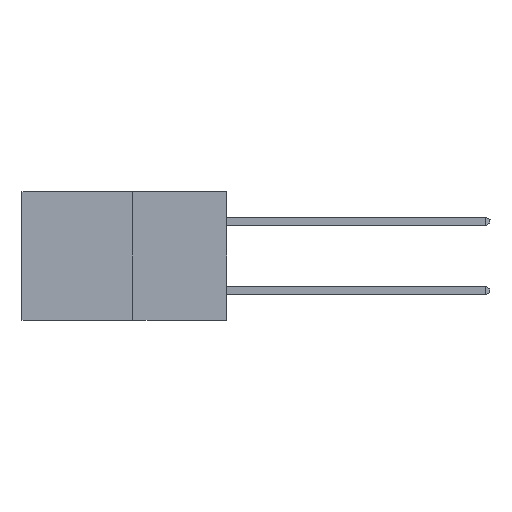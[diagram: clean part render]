
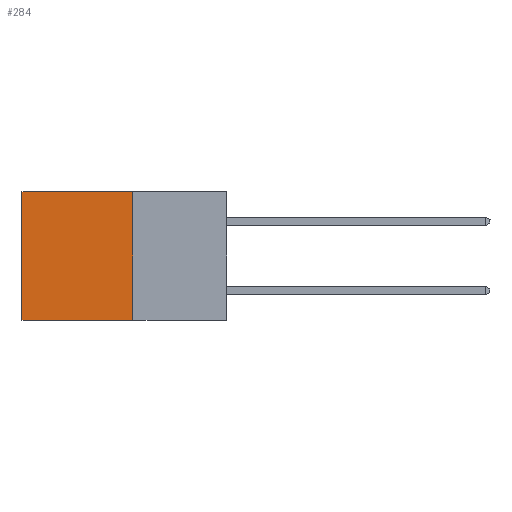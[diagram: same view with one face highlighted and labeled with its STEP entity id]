
A CAD part, left-side view. The second image highlights one B-rep face of the part: STEP entity #284.
In plain terms, the highlighted planar face has unit normal (-1, 0, 0).
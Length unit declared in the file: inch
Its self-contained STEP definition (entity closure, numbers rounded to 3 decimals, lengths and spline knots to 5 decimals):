
#87 = VERTEX_POINT ( 'NONE', #6287 ) ;
#284 = ADVANCED_FACE ( 'NONE', ( #5875 ), #5725, .F. ) ;
#483 = EDGE_LOOP ( 'NONE', ( #6518, #4059, #4269, #2245 ) ) ;
#1002 = LINE ( 'NONE', #7193, #3071 ) ;
#1173 = EDGE_CURVE ( 'NONE', #4882, #4775, #4418, .T. ) ;
#1178 = LINE ( 'NONE', #4783, #8366 ) ;
#1211 = VECTOR ( 'NONE', #1997, 39.37008 ) ;
#1997 = DIRECTION ( 'NONE',  ( 0., 0., -1. ) ) ;
#2168 = DIRECTION ( 'NONE',  ( 0., 1., 0. ) ) ;
#2245 = ORIENTED_EDGE ( 'NONE', *, *, #6026, .T. ) ;
#2585 = CARTESIAN_POINT ( 'NONE',  ( 0.277, 0.27, -0.37 ) ) ;
#2614 = VECTOR ( 'NONE', #2168, 39.37008 ) ;
#2670 = EDGE_CURVE ( 'NONE', #8515, #4882, #1178, .T. ) ;
#2672 = DIRECTION ( 'NONE',  ( 0., 0., -1. ) ) ;
#3006 = DIRECTION ( 'NONE',  ( 0., 1., 0. ) ) ;
#3071 = VECTOR ( 'NONE', #3006, 39.37008 ) ;
#4048 = CARTESIAN_POINT ( 'NONE',  ( 0.277, 0.59, -0.37 ) ) ;
#4059 = ORIENTED_EDGE ( 'NONE', *, *, #1173, .F. ) ;
#4269 = ORIENTED_EDGE ( 'NONE', *, *, #2670, .F. ) ;
#4418 = LINE ( 'NONE', #6122, #2614 ) ;
#4775 = VERTEX_POINT ( 'NONE', #4048 ) ;
#4783 = CARTESIAN_POINT ( 'NONE',  ( 0.277, 0.27, -0.37 ) ) ;
#4882 = VERTEX_POINT ( 'NONE', #2585 ) ;
#4930 = CARTESIAN_POINT ( 'NONE',  ( 0.277, 0.27, 0. ) ) ;
#5408 = CARTESIAN_POINT ( 'NONE',  ( 0.277, 0.59, -0.37 ) ) ;
#5725 = PLANE ( 'NONE',  #7421 ) ;
#5872 = DIRECTION ( 'NONE',  ( 0., 0., -1. ) ) ;
#5875 = FACE_OUTER_BOUND ( 'NONE', #483, .T. ) ;
#6026 = EDGE_CURVE ( 'NONE', #8515, #87, #1002, .T. ) ;
#6033 = CARTESIAN_POINT ( 'NONE',  ( 0.277, 0.27, -0.37 ) ) ;
#6122 = CARTESIAN_POINT ( 'NONE',  ( 0.277, 0.27, -0.37 ) ) ;
#6287 = CARTESIAN_POINT ( 'NONE',  ( 0.277, 0.59, 0. ) ) ;
#6518 = ORIENTED_EDGE ( 'NONE', *, *, #7820, .T. ) ;
#6760 = LINE ( 'NONE', #5408, #1211 ) ;
#7193 = CARTESIAN_POINT ( 'NONE',  ( 0.277, 0.27, 0. ) ) ;
#7421 = AXIS2_PLACEMENT_3D ( 'NONE', #6033, #8270, #2672 ) ;
#7820 = EDGE_CURVE ( 'NONE', #87, #4775, #6760, .T. ) ;
#8270 = DIRECTION ( 'NONE',  ( 1., 0., 0. ) ) ;
#8366 = VECTOR ( 'NONE', #5872, 39.37008 ) ;
#8515 = VERTEX_POINT ( 'NONE', #4930 ) ;
